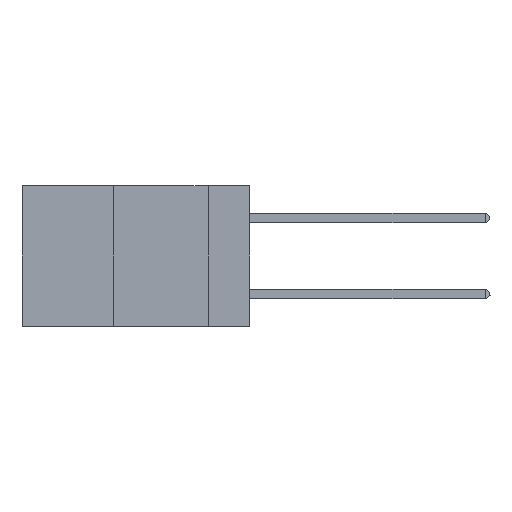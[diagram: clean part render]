
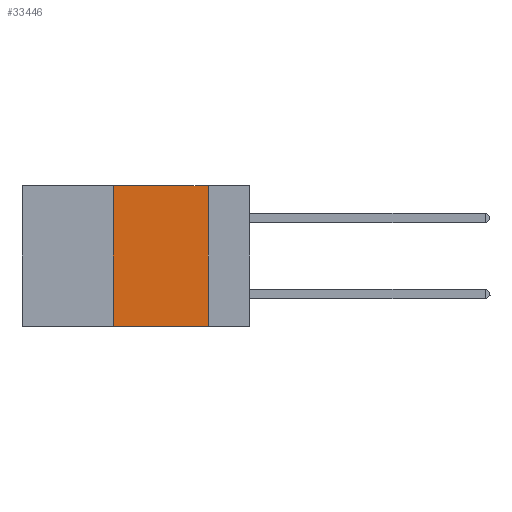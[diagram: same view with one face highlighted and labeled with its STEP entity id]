
A CAD part, left-side view. The second image highlights one B-rep face of the part: STEP entity #33446.
In plain terms, the highlighted planar face has unit normal (-1, 0, 0).
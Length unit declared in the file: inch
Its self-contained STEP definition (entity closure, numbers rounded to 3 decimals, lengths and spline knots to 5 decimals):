
#1010 = CARTESIAN_POINT ( 'NONE',  ( 0., 0.36, 0. ) ) ;
#2767 = CARTESIAN_POINT ( 'NONE',  ( 0., 0.36, -0.37 ) ) ;
#2853 = ORIENTED_EDGE ( 'NONE', *, *, #23401, .T. ) ;
#3773 = PLANE ( 'NONE',  #23393 ) ;
#5104 = ORIENTED_EDGE ( 'NONE', *, *, #13842, .F. ) ;
#6236 = LINE ( 'NONE', #12001, #31935 ) ;
#6366 = DIRECTION ( 'NONE',  ( 1., 0., 0. ) ) ;
#6507 = DIRECTION ( 'NONE',  ( 0., -1., 0. ) ) ;
#6912 = CARTESIAN_POINT ( 'NONE',  ( 0., 0.6, 0. ) ) ;
#9154 = VERTEX_POINT ( 'NONE', #2767 ) ;
#9344 = DIRECTION ( 'NONE',  ( 0., 0., -1. ) ) ;
#10694 = VERTEX_POINT ( 'NONE', #34277 ) ;
#11756 = FACE_OUTER_BOUND ( 'NONE', #18069, .T. ) ;
#12001 = CARTESIAN_POINT ( 'NONE',  ( 0., 0.11, 0. ) ) ;
#12355 = DIRECTION ( 'NONE',  ( 0., 0., -1. ) ) ;
#13842 = EDGE_CURVE ( 'NONE', #32255, #36059, #23303, .T. ) ;
#17544 = CARTESIAN_POINT ( 'NONE',  ( 0., 0.6, 0. ) ) ;
#17602 = DIRECTION ( 'NONE',  ( 0., 0., 1. ) ) ;
#18069 = EDGE_LOOP ( 'NONE', ( #31569, #5104, #35758, #2853 ) ) ;
#19728 = EDGE_CURVE ( 'NONE', #9154, #32255, #29337, .T. ) ;
#21383 = VECTOR ( 'NONE', #32232, 39.37008 ) ;
#22471 = EDGE_CURVE ( 'NONE', #36059, #10694, #6236, .T. ) ;
#23274 = LINE ( 'NONE', #29417, #24831 ) ;
#23303 = LINE ( 'NONE', #6912, #21383 ) ;
#23393 = AXIS2_PLACEMENT_3D ( 'NONE', #17544, #6366, #9344 ) ;
#23401 = EDGE_CURVE ( 'NONE', #9154, #10694, #23274, .T. ) ;
#24831 = VECTOR ( 'NONE', #6507, 39.37008 ) ;
#26136 = CARTESIAN_POINT ( 'NONE',  ( 0., 0.11, 0. ) ) ;
#29337 = LINE ( 'NONE', #1010, #31111 ) ;
#29417 = CARTESIAN_POINT ( 'NONE',  ( 0., 0.6, -0.37 ) ) ;
#31111 = VECTOR ( 'NONE', #17602, 39.37008 ) ;
#31569 = ORIENTED_EDGE ( 'NONE', *, *, #22471, .F. ) ;
#31697 = CARTESIAN_POINT ( 'NONE',  ( 0., 0.36, 0. ) ) ;
#31935 = VECTOR ( 'NONE', #12355, 39.37008 ) ;
#32232 = DIRECTION ( 'NONE',  ( 0., -1., 0. ) ) ;
#32255 = VERTEX_POINT ( 'NONE', #31697 ) ;
#33446 = ADVANCED_FACE ( 'NONE', ( #11756 ), #3773, .F. ) ;
#34277 = CARTESIAN_POINT ( 'NONE',  ( 0., 0.11, -0.37 ) ) ;
#35758 = ORIENTED_EDGE ( 'NONE', *, *, #19728, .F. ) ;
#36059 = VERTEX_POINT ( 'NONE', #26136 ) ;
